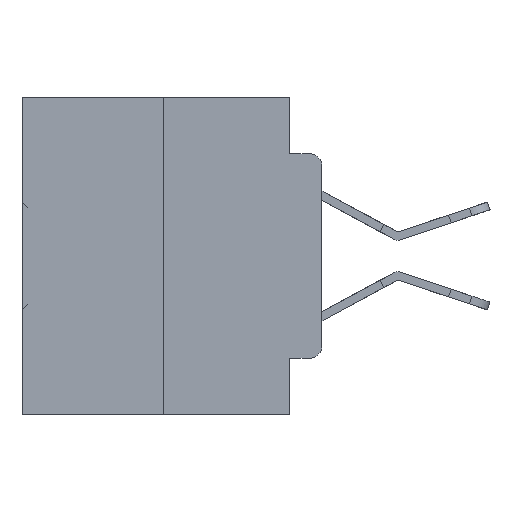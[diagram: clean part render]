
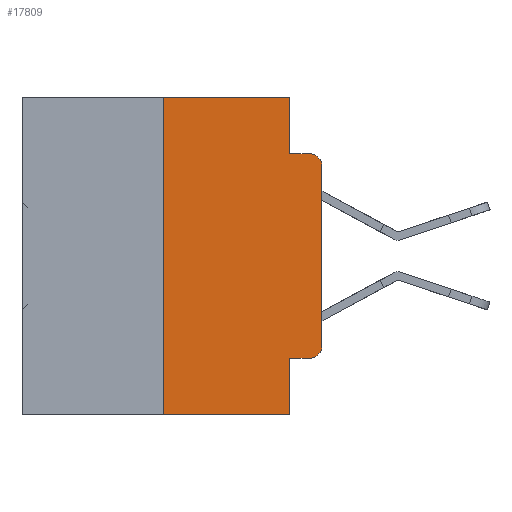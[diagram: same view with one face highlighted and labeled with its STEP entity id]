
A CAD part, left-side view. The second image highlights one B-rep face of the part: STEP entity #17809.
In plain terms, the highlighted planar face has unit normal (-1, 0, 0).
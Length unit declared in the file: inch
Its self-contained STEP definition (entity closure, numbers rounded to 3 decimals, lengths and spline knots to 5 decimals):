
#344 = CARTESIAN_POINT ( 'NONE',  ( 0., 0.051, 0. ) ) ;
#387 = VECTOR ( 'NONE', #21043, 39.37008 ) ;
#554 = LINE ( 'NONE', #24118, #387 ) ;
#1679 = CARTESIAN_POINT ( 'NONE',  ( 0., 0.051, -0.4115 ) ) ;
#1752 = ORIENTED_EDGE ( 'NONE', *, *, #9671, .F. ) ;
#1812 = VERTEX_POINT ( 'NONE', #21220 ) ;
#2004 = AXIS2_PLACEMENT_3D ( 'NONE', #30091, #27449, #3854 ) ;
#2578 = CARTESIAN_POINT ( 'NONE',  ( 0., 0.051, -0.4115 ) ) ;
#2895 = EDGE_CURVE ( 'NONE', #29712, #12201, #554, .T. ) ;
#3854 = DIRECTION ( 'NONE',  ( 0., 0., -1. ) ) ;
#4679 = CARTESIAN_POINT ( 'NONE',  ( 0., 0.051, 0. ) ) ;
#4997 = EDGE_CURVE ( 'NONE', #25620, #1812, #29530, .T. ) ;
#5531 = VECTOR ( 'NONE', #17694, 39.37008 ) ;
#5684 = VERTEX_POINT ( 'NONE', #30396 ) ;
#5934 = ORIENTED_EDGE ( 'NONE', *, *, #11943, .T. ) ;
#7106 = EDGE_LOOP ( 'NONE', ( #34514, #19222, #30459, #11266, #34076, #16142, #29929, #1752, #5934, #26317 ) ) ;
#7428 = LINE ( 'NONE', #13324, #11063 ) ;
#7506 = CIRCLE ( 'NONE', #18428, 0.02 ) ;
#8412 = CARTESIAN_POINT ( 'NONE',  ( 0., 0., -0.3915 ) ) ;
#8553 = DIRECTION ( 'NONE',  ( -1., 0., 0. ) ) ;
#8780 = DIRECTION ( 'NONE',  ( 0., 0., 1. ) ) ;
#8889 = CARTESIAN_POINT ( 'NONE',  ( 0., 0.02, -0.1085 ) ) ;
#9048 = CARTESIAN_POINT ( 'NONE',  ( 0., 0.051, -0.5 ) ) ;
#9371 = PLANE ( 'NONE',  #2004 ) ;
#9414 = VERTEX_POINT ( 'NONE', #24704 ) ;
#9671 = EDGE_CURVE ( 'NONE', #12917, #35723, #14964, .T. ) ;
#11055 = EDGE_CURVE ( 'NONE', #9414, #12201, #7506, .T. ) ;
#11063 = VECTOR ( 'NONE', #36748, 39.37008 ) ;
#11266 = ORIENTED_EDGE ( 'NONE', *, *, #35995, .F. ) ;
#11943 = EDGE_CURVE ( 'NONE', #12917, #26976, #23080, .T. ) ;
#12201 = VERTEX_POINT ( 'NONE', #19424 ) ;
#12917 = VERTEX_POINT ( 'NONE', #1679 ) ;
#13324 = CARTESIAN_POINT ( 'NONE',  ( 0., 0.25, 0. ) ) ;
#13421 = EDGE_CURVE ( 'NONE', #21604, #9414, #13592, .T. ) ;
#13592 = LINE ( 'NONE', #23422, #34014 ) ;
#14053 = CARTESIAN_POINT ( 'NONE',  ( 0., 0.473, -0.5 ) ) ;
#14964 = LINE ( 'NONE', #344, #28909 ) ;
#15548 = EDGE_CURVE ( 'NONE', #5684, #35723, #34781, .T. ) ;
#16142 = ORIENTED_EDGE ( 'NONE', *, *, #31829, .F. ) ;
#16715 = DIRECTION ( 'NONE',  ( 0., -1., 0. ) ) ;
#17694 = DIRECTION ( 'NONE',  ( 0., -1., 0. ) ) ;
#17809 = ADVANCED_FACE ( 'NONE', ( #29723 ), #9371, .F. ) ;
#18428 = AXIS2_PLACEMENT_3D ( 'NONE', #8889, #23152, #32273 ) ;
#19108 = LINE ( 'NONE', #4679, #32203 ) ;
#19222 = ORIENTED_EDGE ( 'NONE', *, *, #11055, .T. ) ;
#19225 = AXIS2_PLACEMENT_3D ( 'NONE', #34611, #8553, #23393 ) ;
#19424 = CARTESIAN_POINT ( 'NONE',  ( 0., 0.02, -0.0885 ) ) ;
#19468 = VECTOR ( 'NONE', #16715, 39.37008 ) ;
#20691 = CARTESIAN_POINT ( 'NONE',  ( 0., 0.25, 0. ) ) ;
#21043 = DIRECTION ( 'NONE',  ( 0., -1., 0. ) ) ;
#21101 = CARTESIAN_POINT ( 'NONE',  ( 0., 0.473, 0. ) ) ;
#21220 = CARTESIAN_POINT ( 'NONE',  ( 0., 0.051, 0. ) ) ;
#21604 = VERTEX_POINT ( 'NONE', #8412 ) ;
#23080 = LINE ( 'NONE', #2578, #24816 ) ;
#23152 = DIRECTION ( 'NONE',  ( -1., 0., 0. ) ) ;
#23354 = EDGE_CURVE ( 'NONE', #26976, #21604, #27152, .T. ) ;
#23393 = DIRECTION ( 'NONE',  ( 0., 0., -1. ) ) ;
#23422 = CARTESIAN_POINT ( 'NONE',  ( 0., 0., 0. ) ) ;
#24118 = CARTESIAN_POINT ( 'NONE',  ( 0., 0.051, -0.0885 ) ) ;
#24260 = DIRECTION ( 'NONE',  ( 0., 0., -1. ) ) ;
#24528 = CARTESIAN_POINT ( 'NONE',  ( 0., 0.02, -0.4115 ) ) ;
#24704 = CARTESIAN_POINT ( 'NONE',  ( 0., 0., -0.1085 ) ) ;
#24816 = VECTOR ( 'NONE', #31473, 39.37008 ) ;
#25620 = VERTEX_POINT ( 'NONE', #20691 ) ;
#26317 = ORIENTED_EDGE ( 'NONE', *, *, #23354, .T. ) ;
#26976 = VERTEX_POINT ( 'NONE', #24528 ) ;
#27152 = CIRCLE ( 'NONE', #19225, 0.02 ) ;
#27449 = DIRECTION ( 'NONE',  ( 1., 0., 0. ) ) ;
#28909 = VECTOR ( 'NONE', #35120, 39.37008 ) ;
#29530 = LINE ( 'NONE', #21101, #5531 ) ;
#29712 = VERTEX_POINT ( 'NONE', #31491 ) ;
#29723 = FACE_OUTER_BOUND ( 'NONE', #7106, .T. ) ;
#29929 = ORIENTED_EDGE ( 'NONE', *, *, #15548, .T. ) ;
#30091 = CARTESIAN_POINT ( 'NONE',  ( 0., 0.473, 0. ) ) ;
#30396 = CARTESIAN_POINT ( 'NONE',  ( 0., 0.25, -0.5 ) ) ;
#30459 = ORIENTED_EDGE ( 'NONE', *, *, #2895, .F. ) ;
#31473 = DIRECTION ( 'NONE',  ( 0., -1., 0. ) ) ;
#31491 = CARTESIAN_POINT ( 'NONE',  ( 0., 0.051, -0.0885 ) ) ;
#31829 = EDGE_CURVE ( 'NONE', #5684, #25620, #7428, .T. ) ;
#32203 = VECTOR ( 'NONE', #24260, 39.37008 ) ;
#32273 = DIRECTION ( 'NONE',  ( 0., 0., -1. ) ) ;
#34014 = VECTOR ( 'NONE', #8780, 39.37008 ) ;
#34076 = ORIENTED_EDGE ( 'NONE', *, *, #4997, .F. ) ;
#34514 = ORIENTED_EDGE ( 'NONE', *, *, #13421, .T. ) ;
#34611 = CARTESIAN_POINT ( 'NONE',  ( 0., 0.02, -0.3915 ) ) ;
#34781 = LINE ( 'NONE', #14053, #19468 ) ;
#35120 = DIRECTION ( 'NONE',  ( 0., 0., -1. ) ) ;
#35723 = VERTEX_POINT ( 'NONE', #9048 ) ;
#35995 = EDGE_CURVE ( 'NONE', #1812, #29712, #19108, .T. ) ;
#36748 = DIRECTION ( 'NONE',  ( 0., 0., 1. ) ) ;
